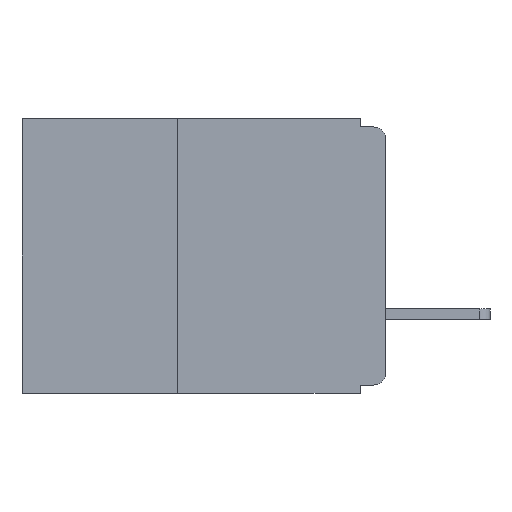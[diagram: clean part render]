
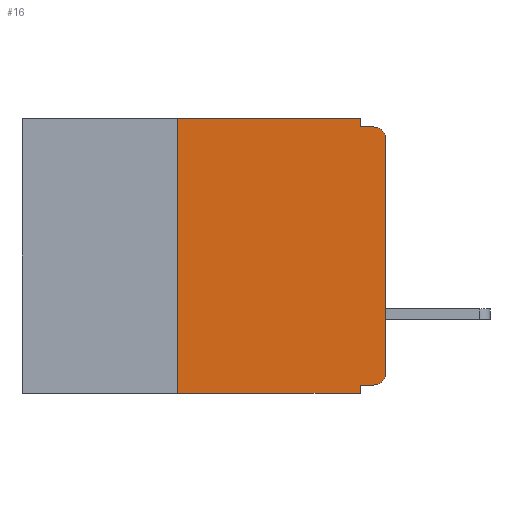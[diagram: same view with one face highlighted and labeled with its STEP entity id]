
A CAD part, left-side view. The second image highlights one B-rep face of the part: STEP entity #16.
In plain terms, the highlighted planar face has unit normal (-1, 0, 0).
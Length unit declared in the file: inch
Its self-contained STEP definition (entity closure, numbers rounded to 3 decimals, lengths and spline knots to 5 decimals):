
#16 = ADVANCED_FACE ( 'NONE', ( #1555 ), #13628, .F. ) ;
#438 = ORIENTED_EDGE ( 'NONE', *, *, #17997, .T. ) ;
#471 = DIRECTION ( 'NONE',  ( -1., 0., 0. ) ) ;
#935 = ORIENTED_EDGE ( 'NONE', *, *, #4303, .F. ) ;
#1017 = CARTESIAN_POINT ( 'NONE',  ( 0., 0.25, -0.33 ) ) ;
#1275 = VECTOR ( 'NONE', #9321, 39.37008 ) ;
#1293 = AXIS2_PLACEMENT_3D ( 'NONE', #13578, #13487, #14124 ) ;
#1555 = FACE_OUTER_BOUND ( 'NONE', #11377, .T. ) ;
#1623 = VERTEX_POINT ( 'NONE', #5076 ) ;
#1760 = LINE ( 'NONE', #10515, #18043 ) ;
#2185 = VERTEX_POINT ( 'NONE', #15906 ) ;
#2884 = CIRCLE ( 'NONE', #14412, 0.015 ) ;
#3224 = ORIENTED_EDGE ( 'NONE', *, *, #9596, .F. ) ;
#3251 = AXIS2_PLACEMENT_3D ( 'NONE', #10062, #471, #11623 ) ;
#3713 = ORIENTED_EDGE ( 'NONE', *, *, #10960, .F. ) ;
#3746 = DIRECTION ( 'NONE',  ( 0., 1., 0. ) ) ;
#3801 = CARTESIAN_POINT ( 'NONE',  ( 0., 0.437, -0.33 ) ) ;
#4011 = CARTESIAN_POINT ( 'NONE',  ( 0., 0., -0.025 ) ) ;
#4303 = EDGE_CURVE ( 'NONE', #9690, #6831, #5568, .T. ) ;
#5076 = CARTESIAN_POINT ( 'NONE',  ( 0., 0.25, -0.33 ) ) ;
#5332 = CARTESIAN_POINT ( 'NONE',  ( 0., 0., -0.01 ) ) ;
#5501 = VECTOR ( 'NONE', #10760, 39.37008 ) ;
#5568 = LINE ( 'NONE', #17094, #1275 ) ;
#5740 = ORIENTED_EDGE ( 'NONE', *, *, #13132, .F. ) ;
#5999 = LINE ( 'NONE', #16975, #5501 ) ;
#6160 = CARTESIAN_POINT ( 'NONE',  ( 0., 0., -0.305 ) ) ;
#6831 = VERTEX_POINT ( 'NONE', #19010 ) ;
#7058 = LINE ( 'NONE', #12436, #14939 ) ;
#7173 = VERTEX_POINT ( 'NONE', #10673 ) ;
#7254 = DIRECTION ( 'NONE',  ( -1., 0., 0. ) ) ;
#7417 = CARTESIAN_POINT ( 'NONE',  ( 0., 0.031, -0.01 ) ) ;
#7859 = CARTESIAN_POINT ( 'NONE',  ( 0., 0.031, 0. ) ) ;
#7937 = EDGE_CURVE ( 'NONE', #9058, #2185, #2884, .T. ) ;
#7939 = ORIENTED_EDGE ( 'NONE', *, *, #17057, .F. ) ;
#8547 = CARTESIAN_POINT ( 'NONE',  ( 0., 0., -0.32 ) ) ;
#9058 = VERTEX_POINT ( 'NONE', #4011 ) ;
#9163 = VERTEX_POINT ( 'NONE', #7417 ) ;
#9321 = DIRECTION ( 'NONE',  ( 0., 0., -1. ) ) ;
#9596 = EDGE_CURVE ( 'NONE', #9163, #2185, #20008, .T. ) ;
#9690 = VERTEX_POINT ( 'NONE', #19560 ) ;
#9950 = ORIENTED_EDGE ( 'NONE', *, *, #13772, .T. ) ;
#10062 = CARTESIAN_POINT ( 'NONE',  ( 0., 0.015, -0.305 ) ) ;
#10112 = DIRECTION ( 'NONE',  ( 0., -1., 0. ) ) ;
#10515 = CARTESIAN_POINT ( 'NONE',  ( 0., 0.437, 0. ) ) ;
#10673 = CARTESIAN_POINT ( 'NONE',  ( 0., 0.25, 0. ) ) ;
#10685 = ORIENTED_EDGE ( 'NONE', *, *, #13400, .T. ) ;
#10760 = DIRECTION ( 'NONE',  ( 0., 0., 1. ) ) ;
#10960 = EDGE_CURVE ( 'NONE', #12904, #9163, #7058, .T. ) ;
#10966 = VERTEX_POINT ( 'NONE', #6160 ) ;
#11377 = EDGE_LOOP ( 'NONE', ( #10685, #15326, #3224, #3713, #7939, #16801, #438, #935, #5740, #9950 ) ) ;
#11623 = DIRECTION ( 'NONE',  ( 0., 0., -1. ) ) ;
#11913 = LINE ( 'NONE', #3801, #15103 ) ;
#12085 = DIRECTION ( 'NONE',  ( 0., -1., 0. ) ) ;
#12157 = DIRECTION ( 'NONE',  ( 0., 0., 1. ) ) ;
#12436 = CARTESIAN_POINT ( 'NONE',  ( 0., 0.031, 0. ) ) ;
#12904 = VERTEX_POINT ( 'NONE', #7859 ) ;
#13132 = EDGE_CURVE ( 'NONE', #13528, #9690, #14842, .T. ) ;
#13400 = EDGE_CURVE ( 'NONE', #10966, #9058, #5999, .T. ) ;
#13487 = DIRECTION ( 'NONE',  ( 1., 0., 0. ) ) ;
#13528 = VERTEX_POINT ( 'NONE', #18808 ) ;
#13578 = CARTESIAN_POINT ( 'NONE',  ( 0., 0.437, 0. ) ) ;
#13628 = PLANE ( 'NONE',  #1293 ) ;
#13772 = EDGE_CURVE ( 'NONE', #13528, #10966, #16317, .T. ) ;
#14124 = DIRECTION ( 'NONE',  ( 0., 0., -1. ) ) ;
#14412 = AXIS2_PLACEMENT_3D ( 'NONE', #16679, #7254, #18197 ) ;
#14491 = EDGE_CURVE ( 'NONE', #1623, #7173, #19124, .T. ) ;
#14842 = LINE ( 'NONE', #8547, #18905 ) ;
#14859 = DIRECTION ( 'NONE',  ( 0., -1., 0. ) ) ;
#14939 = VECTOR ( 'NONE', #17082, 39.37008 ) ;
#15060 = VECTOR ( 'NONE', #12157, 39.37008 ) ;
#15103 = VECTOR ( 'NONE', #14859, 39.37008 ) ;
#15326 = ORIENTED_EDGE ( 'NONE', *, *, #7937, .T. ) ;
#15479 = VECTOR ( 'NONE', #10112, 39.37008 ) ;
#15906 = CARTESIAN_POINT ( 'NONE',  ( 0., 0.015, -0.01 ) ) ;
#16317 = CIRCLE ( 'NONE', #3251, 0.015 ) ;
#16679 = CARTESIAN_POINT ( 'NONE',  ( 0., 0.015, -0.025 ) ) ;
#16801 = ORIENTED_EDGE ( 'NONE', *, *, #14491, .F. ) ;
#16975 = CARTESIAN_POINT ( 'NONE',  ( 0., 0., 0. ) ) ;
#17057 = EDGE_CURVE ( 'NONE', #7173, #12904, #1760, .T. ) ;
#17082 = DIRECTION ( 'NONE',  ( 0., 0., -1. ) ) ;
#17094 = CARTESIAN_POINT ( 'NONE',  ( 0., 0.031, -0.33 ) ) ;
#17997 = EDGE_CURVE ( 'NONE', #1623, #6831, #11913, .T. ) ;
#18043 = VECTOR ( 'NONE', #12085, 39.37008 ) ;
#18197 = DIRECTION ( 'NONE',  ( 0., 0., -1. ) ) ;
#18808 = CARTESIAN_POINT ( 'NONE',  ( 0., 0.015, -0.32 ) ) ;
#18905 = VECTOR ( 'NONE', #3746, 39.37008 ) ;
#19010 = CARTESIAN_POINT ( 'NONE',  ( 0., 0.031, -0.33 ) ) ;
#19124 = LINE ( 'NONE', #1017, #15060 ) ;
#19560 = CARTESIAN_POINT ( 'NONE',  ( 0., 0.031, -0.32 ) ) ;
#20008 = LINE ( 'NONE', #5332, #15479 ) ;
